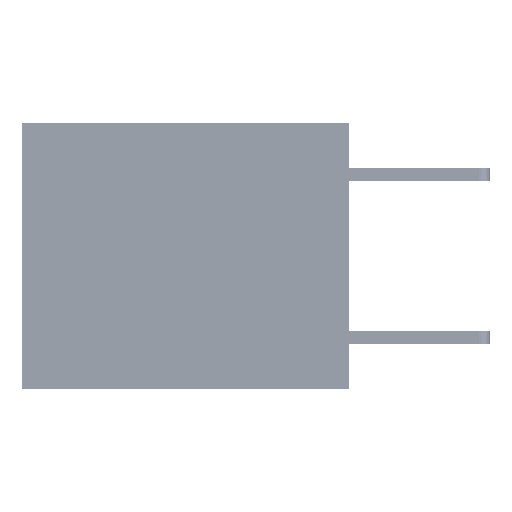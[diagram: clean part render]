
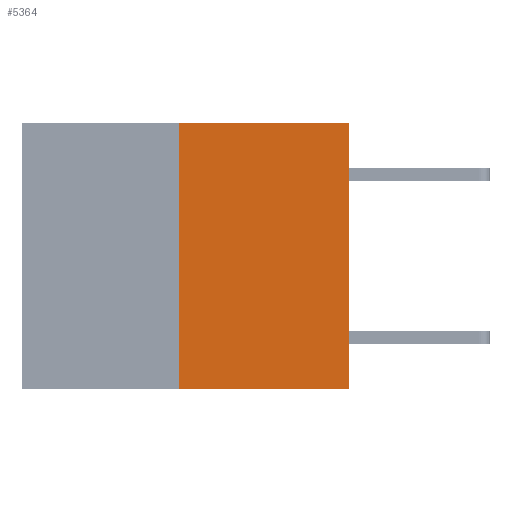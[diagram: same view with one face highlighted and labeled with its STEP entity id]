
A CAD part, left-side view. The second image highlights one B-rep face of the part: STEP entity #5364.
In plain terms, the highlighted planar face has unit normal (-1, 0, 0).
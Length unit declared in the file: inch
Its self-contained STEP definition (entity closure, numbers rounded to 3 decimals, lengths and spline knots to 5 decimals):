
#208 = EDGE_CURVE ( 'NONE', #9759, #12691, #33764, .T. ) ;
#535 = AXIS2_PLACEMENT_3D ( 'NONE', #33720, #17677, #4341 ) ;
#564 = CARTESIAN_POINT ( 'NONE',  ( 0., 0.6, 0. ) ) ;
#1405 = PLANE ( 'NONE',  #535 ) ;
#2485 = CARTESIAN_POINT ( 'NONE',  ( 0., 0.6, -0.49 ) ) ;
#2618 = CARTESIAN_POINT ( 'NONE',  ( 0., 0., 0. ) ) ;
#4341 = DIRECTION ( 'NONE',  ( 0., 0., -1. ) ) ;
#4829 = ORIENTED_EDGE ( 'NONE', *, *, #30602, .T. ) ;
#5364 = ADVANCED_FACE ( 'NONE', ( #19720 ), #1405, .F. ) ;
#7694 = LINE ( 'NONE', #2485, #10172 ) ;
#7968 = DIRECTION ( 'NONE',  ( 0., 0., 1. ) ) ;
#8522 = CARTESIAN_POINT ( 'NONE',  ( 0., 0.312, -0.49 ) ) ;
#8891 = ORIENTED_EDGE ( 'NONE', *, *, #208, .F. ) ;
#8993 = LINE ( 'NONE', #20635, #22067 ) ;
#9734 = EDGE_CURVE ( 'NONE', #31913, #16265, #7694, .T. ) ;
#9759 = VERTEX_POINT ( 'NONE', #18443 ) ;
#10172 = VECTOR ( 'NONE', #31866, 39.37008 ) ;
#11105 = LINE ( 'NONE', #13293, #26698 ) ;
#11882 = VECTOR ( 'NONE', #30315, 39.37008 ) ;
#12691 = VERTEX_POINT ( 'NONE', #2618 ) ;
#13293 = CARTESIAN_POINT ( 'NONE',  ( 0., 0.312, -0.49 ) ) ;
#16265 = VERTEX_POINT ( 'NONE', #23109 ) ;
#17385 = EDGE_LOOP ( 'NONE', ( #28961, #17901, #4829, #8891 ) ) ;
#17677 = DIRECTION ( 'NONE',  ( 1., 0., 0. ) ) ;
#17901 = ORIENTED_EDGE ( 'NONE', *, *, #9734, .T. ) ;
#17980 = DIRECTION ( 'NONE',  ( 0., 0., 1. ) ) ;
#18443 = CARTESIAN_POINT ( 'NONE',  ( 0., 0.312, 0. ) ) ;
#19720 = FACE_OUTER_BOUND ( 'NONE', #17385, .T. ) ;
#20635 = CARTESIAN_POINT ( 'NONE',  ( 0., 0., 0. ) ) ;
#22067 = VECTOR ( 'NONE', #17980, 39.37008 ) ;
#23109 = CARTESIAN_POINT ( 'NONE',  ( 0., 0., -0.49 ) ) ;
#26698 = VECTOR ( 'NONE', #7968, 39.37008 ) ;
#28961 = ORIENTED_EDGE ( 'NONE', *, *, #30299, .F. ) ;
#30299 = EDGE_CURVE ( 'NONE', #31913, #9759, #11105, .T. ) ;
#30315 = DIRECTION ( 'NONE',  ( 0., -1., 0. ) ) ;
#30602 = EDGE_CURVE ( 'NONE', #16265, #12691, #8993, .T. ) ;
#31866 = DIRECTION ( 'NONE',  ( 0., -1., 0. ) ) ;
#31913 = VERTEX_POINT ( 'NONE', #8522 ) ;
#33720 = CARTESIAN_POINT ( 'NONE',  ( 0., 0.6, 0. ) ) ;
#33764 = LINE ( 'NONE', #564, #11882 ) ;
